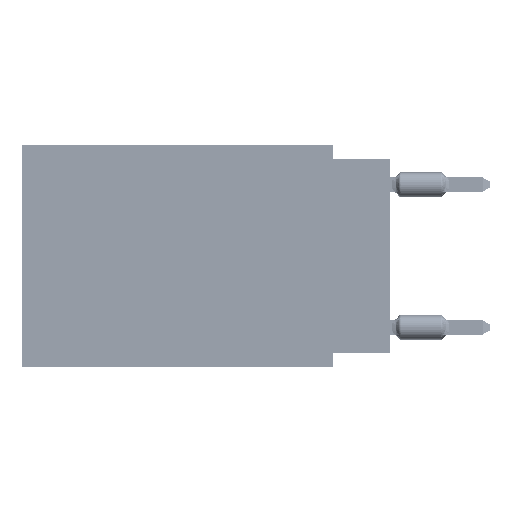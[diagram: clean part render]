
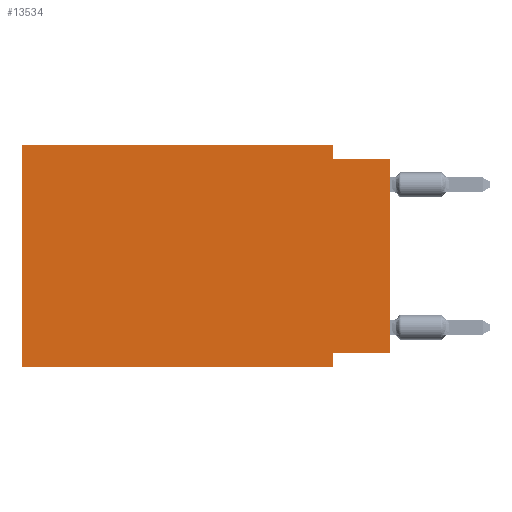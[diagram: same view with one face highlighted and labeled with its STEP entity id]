
A CAD part, left-side view. The second image highlights one B-rep face of the part: STEP entity #13534.
In plain terms, the highlighted planar face has unit normal (-1, 0, 0).
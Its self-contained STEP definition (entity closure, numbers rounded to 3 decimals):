
#594 = ORIENTED_EDGE ( 'NONE', *, *, #27355, .T. ) ;
#712 = AXIS2_PLACEMENT_3D ( 'NONE', #16267, #40937, #34277 ) ;
#3555 = VECTOR ( 'NONE', #42619, 1000. ) ;
#5292 = FACE_OUTER_BOUND ( 'NONE', #14954, .T. ) ;
#7441 = EDGE_CURVE ( 'NONE', #57587, #48432, #49101, .T. ) ;
#10299 = CARTESIAN_POINT ( 'NONE',  ( 0., 2.54, 0. ) ) ;
#10917 = VECTOR ( 'NONE', #32258, 1000. ) ;
#11045 = DIRECTION ( 'NONE',  ( 0., 0., 1. ) ) ;
#11648 = CARTESIAN_POINT ( 'NONE',  ( 0., 16.383, 0. ) ) ;
#11982 = EDGE_CURVE ( 'NONE', #57416, #53052, #70414, .T. ) ;
#12595 = LINE ( 'NONE', #30609, #51630 ) ;
#13534 = ADVANCED_FACE ( 'NONE', ( #5292 ), #22522, .F. ) ;
#14655 = DIRECTION ( 'NONE',  ( 0., -1., 0. ) ) ;
#14954 = EDGE_LOOP ( 'NONE', ( #594, #43305, #72793, #39964, #38992, #63915, #52265, #46532 ) ) ;
#16267 = CARTESIAN_POINT ( 'NONE',  ( 0., 16.383, 0. ) ) ;
#18079 = CARTESIAN_POINT ( 'NONE',  ( 0., 0., -0.635 ) ) ;
#18710 = CARTESIAN_POINT ( 'NONE',  ( 0., 0., -9.271 ) ) ;
#18736 = CARTESIAN_POINT ( 'NONE',  ( 0., 16.383, -9.906 ) ) ;
#19350 = EDGE_CURVE ( 'NONE', #53052, #55027, #74205, .T. ) ;
#19614 = EDGE_CURVE ( 'NONE', #47066, #45004, #61868, .T. ) ;
#22452 = VERTEX_POINT ( 'NONE', #53167 ) ;
#22522 = PLANE ( 'NONE',  #712 ) ;
#27355 = EDGE_CURVE ( 'NONE', #22452, #48432, #12595, .T. ) ;
#29704 = DIRECTION ( 'NONE',  ( 0., 1., 0. ) ) ;
#30609 = CARTESIAN_POINT ( 'NONE',  ( 0., 0., 0. ) ) ;
#31309 = DIRECTION ( 'NONE',  ( 0., 0., -1. ) ) ;
#31489 = CARTESIAN_POINT ( 'NONE',  ( 0., 16.383, 0. ) ) ;
#32258 = DIRECTION ( 'NONE',  ( 0., -1., 0. ) ) ;
#34277 = DIRECTION ( 'NONE',  ( 0., 0., -1. ) ) ;
#37022 = EDGE_CURVE ( 'NONE', #22452, #47066, #48089, .T. ) ;
#38992 = ORIENTED_EDGE ( 'NONE', *, *, #11982, .F. ) ;
#39675 = DIRECTION ( 'NONE',  ( 0., 0., -1. ) ) ;
#39964 = ORIENTED_EDGE ( 'NONE', *, *, #19350, .F. ) ;
#40937 = DIRECTION ( 'NONE',  ( 1., 0., 0. ) ) ;
#42619 = DIRECTION ( 'NONE',  ( 0., -1., 0. ) ) ;
#43305 = ORIENTED_EDGE ( 'NONE', *, *, #7441, .F. ) ;
#43491 = CARTESIAN_POINT ( 'NONE',  ( 0., 2.54, 0. ) ) ;
#45004 = VERTEX_POINT ( 'NONE', #51694 ) ;
#46529 = VECTOR ( 'NONE', #39675, 1000. ) ;
#46532 = ORIENTED_EDGE ( 'NONE', *, *, #37022, .F. ) ;
#46692 = LINE ( 'NONE', #10299, #46529 ) ;
#46873 = DIRECTION ( 'NONE',  ( 0., 0., 1. ) ) ;
#47066 = VERTEX_POINT ( 'NONE', #48494 ) ;
#48089 = LINE ( 'NONE', #18710, #73831 ) ;
#48432 = VERTEX_POINT ( 'NONE', #18079 ) ;
#48494 = CARTESIAN_POINT ( 'NONE',  ( 0., 2.54, -9.271 ) ) ;
#49101 = LINE ( 'NONE', #67161, #10917 ) ;
#49946 = EDGE_CURVE ( 'NONE', #57416, #45004, #72429, .T. ) ;
#51630 = VECTOR ( 'NONE', #11045, 1000. ) ;
#51694 = CARTESIAN_POINT ( 'NONE',  ( 0., 2.54, -9.906 ) ) ;
#52265 = ORIENTED_EDGE ( 'NONE', *, *, #19614, .F. ) ;
#52590 = CARTESIAN_POINT ( 'NONE',  ( 0., 16.383, 0. ) ) ;
#53052 = VERTEX_POINT ( 'NONE', #52590 ) ;
#53167 = CARTESIAN_POINT ( 'NONE',  ( 0., 0., -9.271 ) ) ;
#55027 = VERTEX_POINT ( 'NONE', #43491 ) ;
#57416 = VERTEX_POINT ( 'NONE', #76641 ) ;
#57587 = VERTEX_POINT ( 'NONE', #66076 ) ;
#60926 = EDGE_CURVE ( 'NONE', #55027, #57587, #46692, .T. ) ;
#61480 = CARTESIAN_POINT ( 'NONE',  ( 0., 2.54, -9.906 ) ) ;
#61868 = LINE ( 'NONE', #61480, #64738 ) ;
#63915 = ORIENTED_EDGE ( 'NONE', *, *, #49946, .T. ) ;
#64738 = VECTOR ( 'NONE', #31309, 1000. ) ;
#66076 = CARTESIAN_POINT ( 'NONE',  ( 0., 2.54, -0.635 ) ) ;
#67098 = VECTOR ( 'NONE', #46873, 1000. ) ;
#67161 = CARTESIAN_POINT ( 'NONE',  ( 0., 0., -0.635 ) ) ;
#70414 = LINE ( 'NONE', #11648, #67098 ) ;
#72314 = VECTOR ( 'NONE', #14655, 1000. ) ;
#72429 = LINE ( 'NONE', #18736, #3555 ) ;
#72793 = ORIENTED_EDGE ( 'NONE', *, *, #60926, .F. ) ;
#73831 = VECTOR ( 'NONE', #29704, 1000. ) ;
#74205 = LINE ( 'NONE', #31489, #72314 ) ;
#76641 = CARTESIAN_POINT ( 'NONE',  ( 0., 16.383, -9.906 ) ) ;
